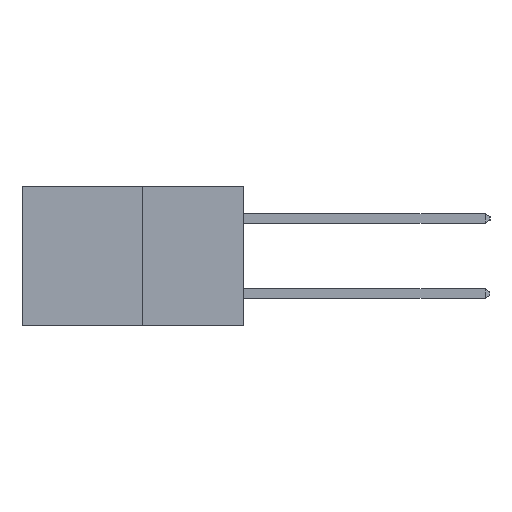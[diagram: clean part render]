
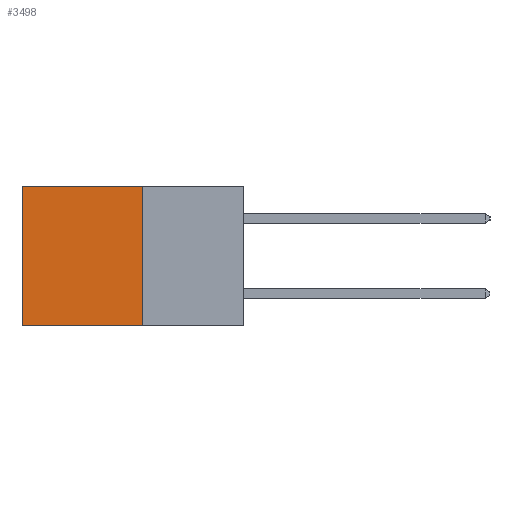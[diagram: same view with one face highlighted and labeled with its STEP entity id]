
A CAD part, left-side view. The second image highlights one B-rep face of the part: STEP entity #3498.
In plain terms, the highlighted planar face has unit normal (-1, 0, 0).
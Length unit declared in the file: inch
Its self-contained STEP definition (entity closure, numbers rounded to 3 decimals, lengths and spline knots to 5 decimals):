
#205 = LINE ( 'NONE', #10852, #11590 ) ;
#206 = AXIS2_PLACEMENT_3D ( 'NONE', #5802, #5788, #5784 ) ;
#413 = LINE ( 'NONE', #452, #5924 ) ;
#452 = CARTESIAN_POINT ( 'NONE',  ( 0.277, 0.27, -0.37 ) ) ;
#694 = EDGE_CURVE ( 'NONE', #9980, #8369, #413, .T. ) ;
#854 = VECTOR ( 'NONE', #1346, 39.37008 ) ;
#1346 = DIRECTION ( 'NONE',  ( 0., 0., -1. ) ) ;
#1819 = EDGE_CURVE ( 'NONE', #7447, #12036, #205, .T. ) ;
#2122 = ORIENTED_EDGE ( 'NONE', *, *, #1819, .T. ) ;
#2352 = CARTESIAN_POINT ( 'NONE',  ( 0.277, 0.27, 0. ) ) ;
#3138 = DIRECTION ( 'NONE',  ( 0., 0., -1. ) ) ;
#3140 = CARTESIAN_POINT ( 'NONE',  ( 0.277, 0.27, -0.37 ) ) ;
#3498 = ADVANCED_FACE ( 'NONE', ( #5340 ), #5837, .F. ) ;
#3723 = LINE ( 'NONE', #3140, #11865 ) ;
#4123 = LINE ( 'NONE', #5729, #854 ) ;
#4401 = EDGE_CURVE ( 'NONE', #7447, #9980, #3723, .T. ) ;
#4648 = DIRECTION ( 'NONE',  ( 0., 1., 0. ) ) ;
#5340 = FACE_OUTER_BOUND ( 'NONE', #11975, .T. ) ;
#5729 = CARTESIAN_POINT ( 'NONE',  ( 0.277, 0.59, -0.37 ) ) ;
#5784 = DIRECTION ( 'NONE',  ( 0., 0., -1. ) ) ;
#5788 = DIRECTION ( 'NONE',  ( 1., 0., 0. ) ) ;
#5802 = CARTESIAN_POINT ( 'NONE',  ( 0.277, 0.27, -0.37 ) ) ;
#5837 = PLANE ( 'NONE',  #206 ) ;
#5924 = VECTOR ( 'NONE', #4648, 39.37008 ) ;
#7447 = VERTEX_POINT ( 'NONE', #2352 ) ;
#8369 = VERTEX_POINT ( 'NONE', #10456 ) ;
#8571 = CARTESIAN_POINT ( 'NONE',  ( 0.277, 0.59, 0. ) ) ;
#9310 = ORIENTED_EDGE ( 'NONE', *, *, #11614, .T. ) ;
#9511 = CARTESIAN_POINT ( 'NONE',  ( 0.277, 0.27, -0.37 ) ) ;
#9980 = VERTEX_POINT ( 'NONE', #9511 ) ;
#10456 = CARTESIAN_POINT ( 'NONE',  ( 0.277, 0.59, -0.37 ) ) ;
#10852 = CARTESIAN_POINT ( 'NONE',  ( 0.277, 0.27, 0. ) ) ;
#11590 = VECTOR ( 'NONE', #12380, 39.37008 ) ;
#11614 = EDGE_CURVE ( 'NONE', #12036, #8369, #4123, .T. ) ;
#11865 = VECTOR ( 'NONE', #3138, 39.37008 ) ;
#11975 = EDGE_LOOP ( 'NONE', ( #9310, #13931, #13454, #2122 ) ) ;
#12036 = VERTEX_POINT ( 'NONE', #8571 ) ;
#12380 = DIRECTION ( 'NONE',  ( 0., 1., 0. ) ) ;
#13454 = ORIENTED_EDGE ( 'NONE', *, *, #4401, .F. ) ;
#13931 = ORIENTED_EDGE ( 'NONE', *, *, #694, .F. ) ;
